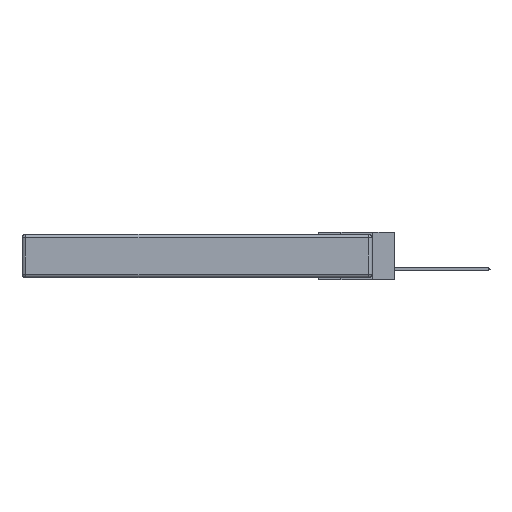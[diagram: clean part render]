
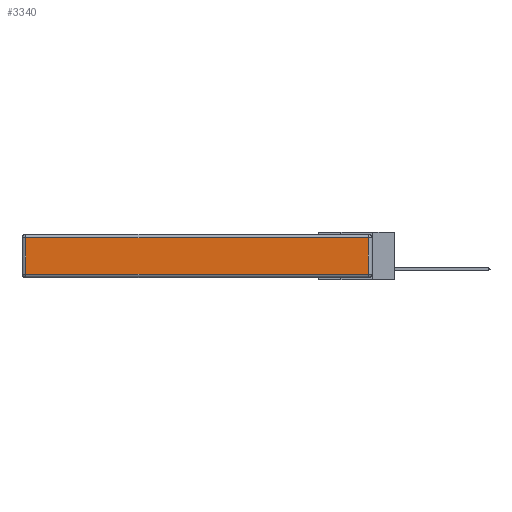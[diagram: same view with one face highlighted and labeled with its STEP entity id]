
A CAD part, left-side view. The second image highlights one B-rep face of the part: STEP entity #3340.
In plain terms, the highlighted planar face has unit normal (-1, 0, 0).
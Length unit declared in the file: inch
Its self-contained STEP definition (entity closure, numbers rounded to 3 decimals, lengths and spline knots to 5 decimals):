
#532 = DIRECTION ( 'NONE',  ( 0., 0., 1. ) ) ;
#860 = LINE ( 'NONE', #18216, #16679 ) ;
#2235 = LINE ( 'NONE', #8397, #6560 ) ;
#2586 = ORIENTED_EDGE ( 'NONE', *, *, #2973, .T. ) ;
#2814 = VERTEX_POINT ( 'NONE', #32688 ) ;
#2973 = EDGE_CURVE ( 'NONE', #8641, #19091, #22615, .T. ) ;
#3070 = ORIENTED_EDGE ( 'NONE', *, *, #28022, .T. ) ;
#3340 = ADVANCED_FACE ( 'NONE', ( #7969 ), #4774, .T. ) ;
#3376 = EDGE_CURVE ( 'NONE', #19091, #6999, #860, .T. ) ;
#4774 = PLANE ( 'NONE',  #27977 ) ;
#4958 = CARTESIAN_POINT ( 'NONE',  ( 0., 0.03, -0.313 ) ) ;
#4986 = DIRECTION ( 'NONE',  ( 0., 0., 1. ) ) ;
#6110 = ORIENTED_EDGE ( 'NONE', *, *, #22548, .T. ) ;
#6560 = VECTOR ( 'NONE', #28286, 39.37008 ) ;
#6999 = VERTEX_POINT ( 'NONE', #24488 ) ;
#7969 = FACE_OUTER_BOUND ( 'NONE', #19934, .T. ) ;
#8397 = CARTESIAN_POINT ( 'NONE',  ( 0., 2.72, -0.343 ) ) ;
#8641 = VERTEX_POINT ( 'NONE', #28269 ) ;
#8865 = CARTESIAN_POINT ( 'NONE',  ( 0., 0., -0.313 ) ) ;
#12383 = DIRECTION ( 'NONE',  ( -1., 0., 0. ) ) ;
#13765 = VECTOR ( 'NONE', #17951, 39.37008 ) ;
#15102 = VECTOR ( 'NONE', #26639, 39.37008 ) ;
#16679 = VECTOR ( 'NONE', #532, 39.37008 ) ;
#17951 = DIRECTION ( 'NONE',  ( 0., 1., 0. ) ) ;
#18216 = CARTESIAN_POINT ( 'NONE',  ( 0., 0.03, -0.343 ) ) ;
#18296 = ORIENTED_EDGE ( 'NONE', *, *, #3376, .T. ) ;
#19091 = VERTEX_POINT ( 'NONE', #4958 ) ;
#19934 = EDGE_LOOP ( 'NONE', ( #2586, #18296, #6110, #3070 ) ) ;
#22548 = EDGE_CURVE ( 'NONE', #6999, #2814, #32698, .T. ) ;
#22615 = LINE ( 'NONE', #8865, #15102 ) ;
#24488 = CARTESIAN_POINT ( 'NONE',  ( 0., 0.03, -0.03 ) ) ;
#26639 = DIRECTION ( 'NONE',  ( 0., -1., 0. ) ) ;
#27502 = CARTESIAN_POINT ( 'NONE',  ( 0., 0., -0.343 ) ) ;
#27977 = AXIS2_PLACEMENT_3D ( 'NONE', #27502, #12383, #4986 ) ;
#27983 = CARTESIAN_POINT ( 'NONE',  ( 0., 2.75, -0.03 ) ) ;
#28022 = EDGE_CURVE ( 'NONE', #2814, #8641, #2235, .T. ) ;
#28269 = CARTESIAN_POINT ( 'NONE',  ( 0., 2.72, -0.313 ) ) ;
#28286 = DIRECTION ( 'NONE',  ( 0., 0., -1. ) ) ;
#32688 = CARTESIAN_POINT ( 'NONE',  ( 0., 2.72, -0.03 ) ) ;
#32698 = LINE ( 'NONE', #27983, #13765 ) ;
